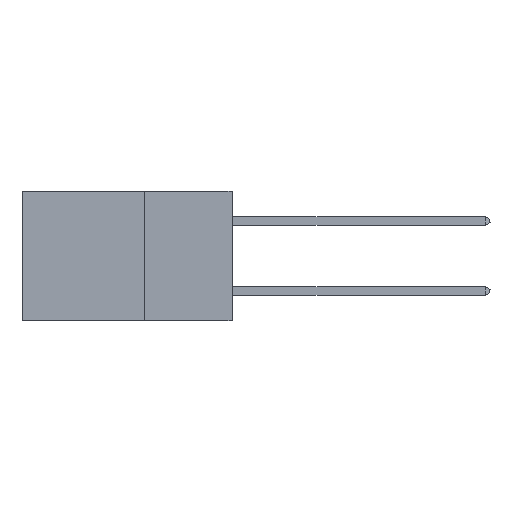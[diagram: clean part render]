
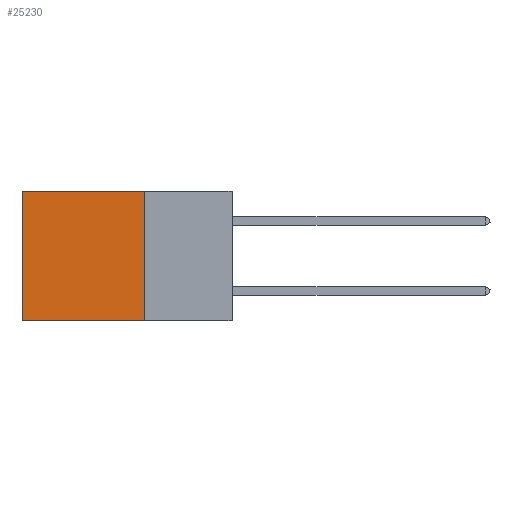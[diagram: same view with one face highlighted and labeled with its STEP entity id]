
A CAD part, left-side view. The second image highlights one B-rep face of the part: STEP entity #25230.
In plain terms, the highlighted planar face has unit normal (-1, 0, 0).
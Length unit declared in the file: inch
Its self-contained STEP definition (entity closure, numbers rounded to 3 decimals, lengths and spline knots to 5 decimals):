
#1750 = VERTEX_POINT ( 'NONE', #26276 ) ;
#2307 = DIRECTION ( 'NONE',  ( 1., 0., 0. ) ) ;
#3782 = ORIENTED_EDGE ( 'NONE', *, *, #18966, .F. ) ;
#3896 = ORIENTED_EDGE ( 'NONE', *, *, #36511, .T. ) ;
#3980 = CARTESIAN_POINT ( 'NONE',  ( 0.2875, 0.25, -0.37 ) ) ;
#6088 = EDGE_CURVE ( 'NONE', #17455, #1750, #31597, .T. ) ;
#8905 = EDGE_LOOP ( 'NONE', ( #3896, #3782, #14221, #38956 ) ) ;
#9038 = CARTESIAN_POINT ( 'NONE',  ( 0.2875, 0.25, 0. ) ) ;
#9314 = CARTESIAN_POINT ( 'NONE',  ( 0.2875, 0.25, 0. ) ) ;
#12708 = DIRECTION ( 'NONE',  ( 0., 1., 0. ) ) ;
#14221 = ORIENTED_EDGE ( 'NONE', *, *, #36093, .F. ) ;
#14650 = CARTESIAN_POINT ( 'NONE',  ( 0.2875, 0.6, 0. ) ) ;
#17455 = VERTEX_POINT ( 'NONE', #33564 ) ;
#18966 = EDGE_CURVE ( 'NONE', #36964, #23124, #37035, .T. ) ;
#19331 = FACE_OUTER_BOUND ( 'NONE', #8905, .T. ) ;
#21075 = VECTOR ( 'NONE', #37379, 39.37008 ) ;
#21776 = CARTESIAN_POINT ( 'NONE',  ( 0.2875, 0.25, 0. ) ) ;
#23124 = VERTEX_POINT ( 'NONE', #25306 ) ;
#23344 = AXIS2_PLACEMENT_3D ( 'NONE', #21776, #2307, #25046 ) ;
#25046 = DIRECTION ( 'NONE',  ( 0., 0., -1. ) ) ;
#25230 = ADVANCED_FACE ( 'NONE', ( #19331 ), #37961, .F. ) ;
#25306 = CARTESIAN_POINT ( 'NONE',  ( 0.2875, 0.6, -0.37 ) ) ;
#26276 = CARTESIAN_POINT ( 'NONE',  ( 0.2875, 0.6, 0. ) ) ;
#28505 = VECTOR ( 'NONE', #12708, 39.37008 ) ;
#30270 = VECTOR ( 'NONE', #38267, 39.37008 ) ;
#31597 = LINE ( 'NONE', #9314, #28505 ) ;
#31850 = CARTESIAN_POINT ( 'NONE',  ( 0.2875, 0.25, -0.37 ) ) ;
#32465 = VECTOR ( 'NONE', #35950, 39.37008 ) ;
#33564 = CARTESIAN_POINT ( 'NONE',  ( 0.2875, 0.25, 0. ) ) ;
#35950 = DIRECTION ( 'NONE',  ( 0., 1., 0. ) ) ;
#36093 = EDGE_CURVE ( 'NONE', #17455, #36964, #40980, .T. ) ;
#36511 = EDGE_CURVE ( 'NONE', #1750, #23124, #37858, .T. ) ;
#36964 = VERTEX_POINT ( 'NONE', #31850 ) ;
#37035 = LINE ( 'NONE', #3980, #32465 ) ;
#37379 = DIRECTION ( 'NONE',  ( 0., 0., -1. ) ) ;
#37858 = LINE ( 'NONE', #14650, #21075 ) ;
#37961 = PLANE ( 'NONE',  #23344 ) ;
#38267 = DIRECTION ( 'NONE',  ( 0., 0., -1. ) ) ;
#38956 = ORIENTED_EDGE ( 'NONE', *, *, #6088, .T. ) ;
#40980 = LINE ( 'NONE', #9038, #30270 ) ;
